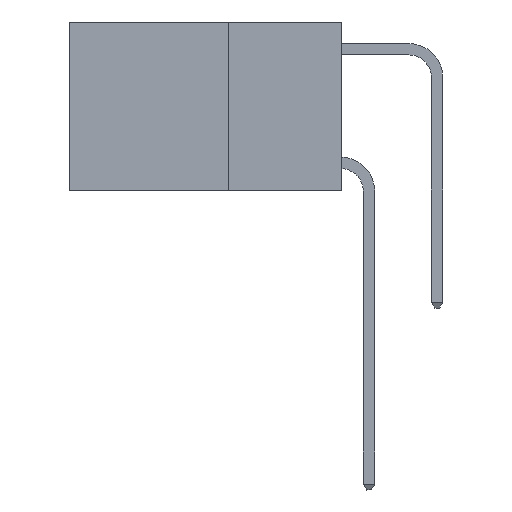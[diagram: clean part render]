
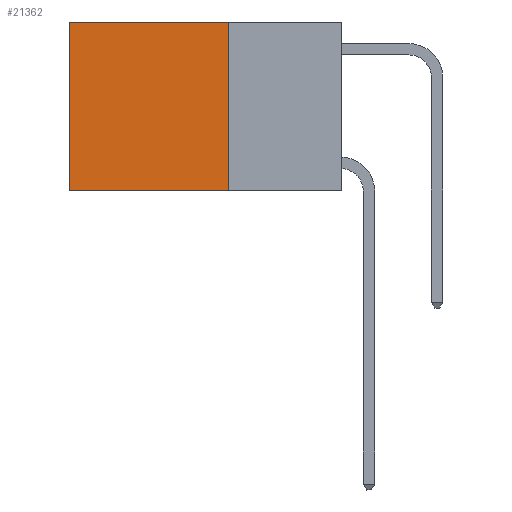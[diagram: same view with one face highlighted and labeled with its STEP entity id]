
A CAD part, left-side view. The second image highlights one B-rep face of the part: STEP entity #21362.
In plain terms, the highlighted planar face has unit normal (-1, 0, 0).
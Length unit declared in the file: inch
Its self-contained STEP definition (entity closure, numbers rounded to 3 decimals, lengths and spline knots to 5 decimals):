
#420 = EDGE_CURVE ( 'NONE', #15298, #8270, #9913, .T. ) ;
#1165 = VERTEX_POINT ( 'NONE', #2458 ) ;
#1778 = FACE_OUTER_BOUND ( 'NONE', #6350, .T. ) ;
#1837 = CARTESIAN_POINT ( 'NONE',  ( 0.2625, 0.25, 0. ) ) ;
#2416 = DIRECTION ( 'NONE',  ( 0., 0., -1. ) ) ;
#2458 = CARTESIAN_POINT ( 'NONE',  ( 0.2625, 0.6, 0. ) ) ;
#2602 = DIRECTION ( 'NONE',  ( 0., 0., -1. ) ) ;
#3593 = DIRECTION ( 'NONE',  ( 0., 1., 0. ) ) ;
#4247 = CARTESIAN_POINT ( 'NONE',  ( 0.2625, 0.25, 0. ) ) ;
#5303 = ORIENTED_EDGE ( 'NONE', *, *, #17519, .T. ) ;
#5922 = VECTOR ( 'NONE', #2602, 39.37008 ) ;
#6350 = EDGE_LOOP ( 'NONE', ( #5303, #14232, #15797, #9920 ) ) ;
#7005 = LINE ( 'NONE', #7702, #5922 ) ;
#7690 = DIRECTION ( 'NONE',  ( 0., 0., -1. ) ) ;
#7702 = CARTESIAN_POINT ( 'NONE',  ( 0.2625, 0.6, 0. ) ) ;
#8270 = VERTEX_POINT ( 'NONE', #15521 ) ;
#9233 = PLANE ( 'NONE',  #15510 ) ;
#9662 = VECTOR ( 'NONE', #7690, 39.37008 ) ;
#9913 = LINE ( 'NONE', #12784, #13417 ) ;
#9920 = ORIENTED_EDGE ( 'NONE', *, *, #11867, .T. ) ;
#10003 = DIRECTION ( 'NONE',  ( 0., 1., 0. ) ) ;
#11568 = EDGE_CURVE ( 'NONE', #18133, #15298, #19269, .T. ) ;
#11867 = EDGE_CURVE ( 'NONE', #18133, #1165, #18460, .T. ) ;
#12708 = DIRECTION ( 'NONE',  ( 1., 0., 0. ) ) ;
#12784 = CARTESIAN_POINT ( 'NONE',  ( 0.2625, 0.25, -0.37 ) ) ;
#13417 = VECTOR ( 'NONE', #10003, 39.37008 ) ;
#14232 = ORIENTED_EDGE ( 'NONE', *, *, #420, .F. ) ;
#15298 = VERTEX_POINT ( 'NONE', #16878 ) ;
#15510 = AXIS2_PLACEMENT_3D ( 'NONE', #19444, #12708, #2416 ) ;
#15521 = CARTESIAN_POINT ( 'NONE',  ( 0.2625, 0.6, -0.37 ) ) ;
#15797 = ORIENTED_EDGE ( 'NONE', *, *, #11568, .F. ) ;
#16878 = CARTESIAN_POINT ( 'NONE',  ( 0.2625, 0.25, -0.37 ) ) ;
#17519 = EDGE_CURVE ( 'NONE', #1165, #8270, #7005, .T. ) ;
#18133 = VERTEX_POINT ( 'NONE', #4247 ) ;
#18460 = LINE ( 'NONE', #1837, #21897 ) ;
#19269 = LINE ( 'NONE', #21325, #9662 ) ;
#19444 = CARTESIAN_POINT ( 'NONE',  ( 0.2625, 0.25, 0. ) ) ;
#21325 = CARTESIAN_POINT ( 'NONE',  ( 0.2625, 0.25, 0. ) ) ;
#21362 = ADVANCED_FACE ( 'NONE', ( #1778 ), #9233, .F. ) ;
#21897 = VECTOR ( 'NONE', #3593, 39.37008 ) ;
